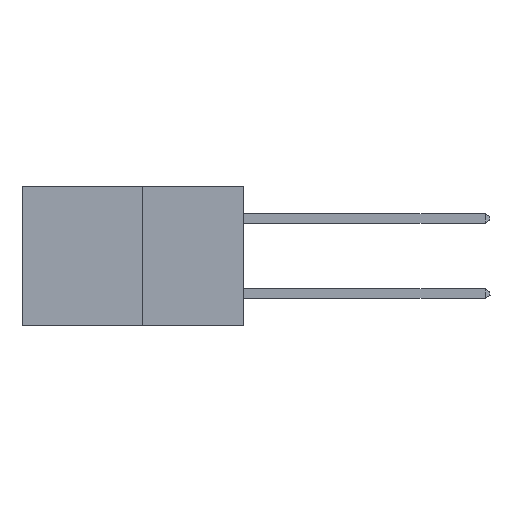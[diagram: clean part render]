
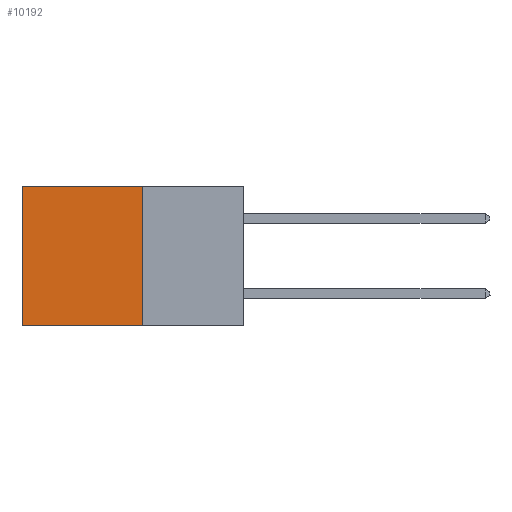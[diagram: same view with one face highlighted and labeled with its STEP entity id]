
A CAD part, left-side view. The second image highlights one B-rep face of the part: STEP entity #10192.
In plain terms, the highlighted planar face has unit normal (-1, 0, 0).
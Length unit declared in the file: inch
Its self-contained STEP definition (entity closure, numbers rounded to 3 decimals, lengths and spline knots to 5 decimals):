
#600 = VECTOR ( 'NONE', #15684, 39.37008 ) ;
#805 = VERTEX_POINT ( 'NONE', #17585 ) ;
#899 = VERTEX_POINT ( 'NONE', #17062 ) ;
#972 = ORIENTED_EDGE ( 'NONE', *, *, #18021, .F. ) ;
#1265 = DIRECTION ( 'NONE',  ( 0., 1., 0. ) ) ;
#1703 = LINE ( 'NONE', #14278, #14333 ) ;
#1992 = ORIENTED_EDGE ( 'NONE', *, *, #2061, .F. ) ;
#2061 = EDGE_CURVE ( 'NONE', #805, #18394, #20216, .T. ) ;
#2525 = ORIENTED_EDGE ( 'NONE', *, *, #3670, .T. ) ;
#3489 = LINE ( 'NONE', #18873, #20087 ) ;
#3670 = EDGE_CURVE ( 'NONE', #805, #899, #1703, .T. ) ;
#3791 = CARTESIAN_POINT ( 'NONE',  ( 0.277, 0.59, -0.37 ) ) ;
#4202 = AXIS2_PLACEMENT_3D ( 'NONE', #10922, #11320, #11226 ) ;
#4472 = EDGE_LOOP ( 'NONE', ( #12338, #972, #1992, #2525 ) ) ;
#6916 = CARTESIAN_POINT ( 'NONE',  ( 0.277, 0.27, -0.37 ) ) ;
#8007 = CARTESIAN_POINT ( 'NONE',  ( 0.277, 0.27, -0.37 ) ) ;
#8566 = VERTEX_POINT ( 'NONE', #3791 ) ;
#8682 = FACE_OUTER_BOUND ( 'NONE', #4472, .T. ) ;
#8924 = DIRECTION ( 'NONE',  ( 0., 0., -1. ) ) ;
#9111 = PLANE ( 'NONE',  #4202 ) ;
#10192 = ADVANCED_FACE ( 'NONE', ( #8682 ), #9111, .F. ) ;
#10922 = CARTESIAN_POINT ( 'NONE',  ( 0.277, 0.27, -0.37 ) ) ;
#11226 = DIRECTION ( 'NONE',  ( 0., 0., -1. ) ) ;
#11320 = DIRECTION ( 'NONE',  ( 1., 0., 0. ) ) ;
#11903 = VECTOR ( 'NONE', #8924, 39.37008 ) ;
#12338 = ORIENTED_EDGE ( 'NONE', *, *, #18080, .T. ) ;
#12424 = CARTESIAN_POINT ( 'NONE',  ( 0.277, 0.27, -0.37 ) ) ;
#14255 = DIRECTION ( 'NONE',  ( 0., 0., -1. ) ) ;
#14278 = CARTESIAN_POINT ( 'NONE',  ( 0.277, 0.27, 0. ) ) ;
#14333 = VECTOR ( 'NONE', #1265, 39.37008 ) ;
#15684 = DIRECTION ( 'NONE',  ( 0., 1., 0. ) ) ;
#17062 = CARTESIAN_POINT ( 'NONE',  ( 0.277, 0.59, 0. ) ) ;
#17585 = CARTESIAN_POINT ( 'NONE',  ( 0.277, 0.27, 0. ) ) ;
#18021 = EDGE_CURVE ( 'NONE', #18394, #8566, #18410, .T. ) ;
#18080 = EDGE_CURVE ( 'NONE', #899, #8566, #3489, .T. ) ;
#18394 = VERTEX_POINT ( 'NONE', #6916 ) ;
#18410 = LINE ( 'NONE', #12424, #600 ) ;
#18873 = CARTESIAN_POINT ( 'NONE',  ( 0.277, 0.59, -0.37 ) ) ;
#20087 = VECTOR ( 'NONE', #14255, 39.37008 ) ;
#20216 = LINE ( 'NONE', #8007, #11903 ) ;
